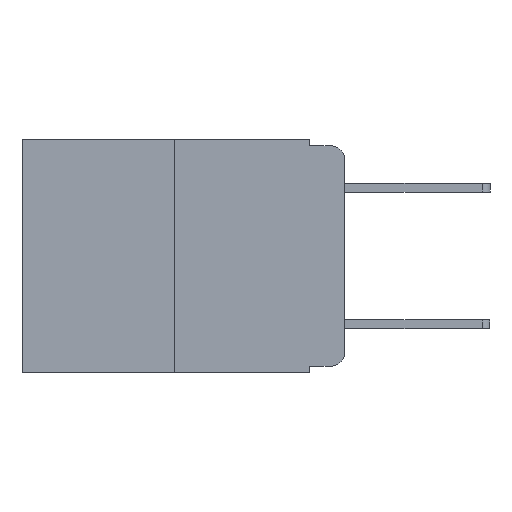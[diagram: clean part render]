
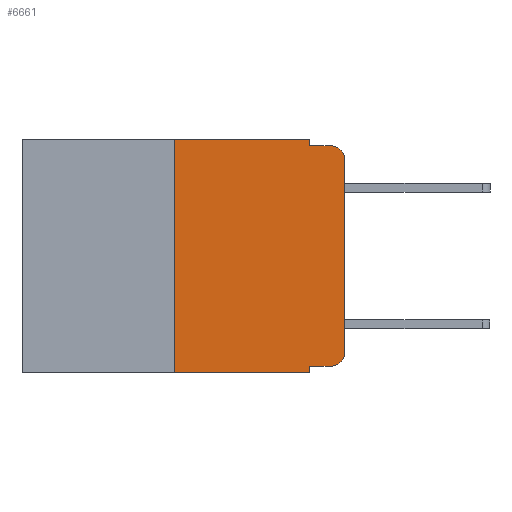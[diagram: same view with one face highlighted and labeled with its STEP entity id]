
A CAD part, left-side view. The second image highlights one B-rep face of the part: STEP entity #6661.
In plain terms, the highlighted planar face has unit normal (-1, 0, 0).
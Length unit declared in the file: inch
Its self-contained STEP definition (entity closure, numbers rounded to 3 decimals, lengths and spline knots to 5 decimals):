
#498 = EDGE_CURVE ( 'NONE', #4194, #19976, #15125, .T. ) ;
#619 = ORIENTED_EDGE ( 'NONE', *, *, #13158, .T. ) ;
#621 = EDGE_CURVE ( 'NONE', #4194, #7882, #17908, .T. ) ;
#713 = CARTESIAN_POINT ( 'NONE',  ( 0., 0.051, -0.01 ) ) ;
#877 = DIRECTION ( 'NONE',  ( 1., 0., 0. ) ) ;
#1221 = CARTESIAN_POINT ( 'NONE',  ( 0., 0.051, -0.343 ) ) ;
#1234 = VECTOR ( 'NONE', #7158, 39.37008 ) ;
#1759 = EDGE_LOOP ( 'NONE', ( #17316, #18535, #5094, #11025, #22263, #22857, #13569, #14815, #619, #7294 ) ) ;
#2315 = VERTEX_POINT ( 'NONE', #12398 ) ;
#2524 = EDGE_CURVE ( 'NONE', #12047, #22004, #4253, .T. ) ;
#2867 = VECTOR ( 'NONE', #16644, 39.37008 ) ;
#3122 = LINE ( 'NONE', #8261, #18510 ) ;
#3480 = DIRECTION ( 'NONE',  ( 0., -1., 0. ) ) ;
#4194 = VERTEX_POINT ( 'NONE', #8887 ) ;
#4246 = VERTEX_POINT ( 'NONE', #22222 ) ;
#4253 = CIRCLE ( 'NONE', #12836, 0.02 ) ;
#4378 = EDGE_CURVE ( 'NONE', #12311, #18752, #13593, .T. ) ;
#5094 = ORIENTED_EDGE ( 'NONE', *, *, #4378, .F. ) ;
#5103 = DIRECTION ( 'NONE',  ( -1., 0., 0. ) ) ;
#5194 = EDGE_CURVE ( 'NONE', #22004, #2315, #16683, .T. ) ;
#5383 = VECTOR ( 'NONE', #17903, 39.37008 ) ;
#5543 = CARTESIAN_POINT ( 'NONE',  ( 0., 0.473, 0. ) ) ;
#6079 = EDGE_CURVE ( 'NONE', #19036, #19976, #25779, .T. ) ;
#6661 = ADVANCED_FACE ( 'NONE', ( #23111 ), #12960, .F. ) ;
#7158 = DIRECTION ( 'NONE',  ( 0., 0., 1. ) ) ;
#7294 = ORIENTED_EDGE ( 'NONE', *, *, #2524, .T. ) ;
#7763 = EDGE_CURVE ( 'NONE', #7882, #4246, #13786, .T. ) ;
#7882 = VERTEX_POINT ( 'NONE', #11914 ) ;
#8009 = CARTESIAN_POINT ( 'NONE',  ( 0., 0.473, -0.343 ) ) ;
#8261 = CARTESIAN_POINT ( 'NONE',  ( 0., 0.051, -0.333 ) ) ;
#8887 = CARTESIAN_POINT ( 'NONE',  ( 0., 0.25, -0.343 ) ) ;
#9467 = CARTESIAN_POINT ( 'NONE',  ( 0., 0.051, -0.333 ) ) ;
#9602 = CARTESIAN_POINT ( 'NONE',  ( 0., 0.051, -0.01 ) ) ;
#9733 = VECTOR ( 'NONE', #19588, 39.37008 ) ;
#9993 = CARTESIAN_POINT ( 'NONE',  ( 0., 0.25, 0. ) ) ;
#10937 = VECTOR ( 'NONE', #14960, 39.37008 ) ;
#11025 = ORIENTED_EDGE ( 'NONE', *, *, #14642, .F. ) ;
#11155 = CARTESIAN_POINT ( 'NONE',  ( 0., 0., -0.313 ) ) ;
#11223 = DIRECTION ( 'NONE',  ( 0., 0., -1. ) ) ;
#11914 = CARTESIAN_POINT ( 'NONE',  ( 0., 0.25, 0. ) ) ;
#12047 = VERTEX_POINT ( 'NONE', #16848 ) ;
#12093 = EDGE_CURVE ( 'NONE', #2315, #18752, #15427, .T. ) ;
#12219 = DIRECTION ( 'NONE',  ( 0., -1., 0. ) ) ;
#12311 = VERTEX_POINT ( 'NONE', #9602 ) ;
#12398 = CARTESIAN_POINT ( 'NONE',  ( 0., 0., -0.03 ) ) ;
#12779 = DIRECTION ( 'NONE',  ( 0., 0., -1. ) ) ;
#12836 = AXIS2_PLACEMENT_3D ( 'NONE', #15555, #18609, #12779 ) ;
#12960 = PLANE ( 'NONE',  #23681 ) ;
#13158 = EDGE_CURVE ( 'NONE', #19036, #12047, #3122, .T. ) ;
#13162 = VECTOR ( 'NONE', #3480, 39.37008 ) ;
#13569 = ORIENTED_EDGE ( 'NONE', *, *, #498, .T. ) ;
#13593 = LINE ( 'NONE', #713, #2867 ) ;
#13786 = LINE ( 'NONE', #5543, #13162 ) ;
#13845 = AXIS2_PLACEMENT_3D ( 'NONE', #17104, #5103, #19094 ) ;
#14642 = EDGE_CURVE ( 'NONE', #4246, #12311, #22182, .T. ) ;
#14815 = ORIENTED_EDGE ( 'NONE', *, *, #6079, .F. ) ;
#14960 = DIRECTION ( 'NONE',  ( 0., 0., -1. ) ) ;
#14984 = DIRECTION ( 'NONE',  ( 0., 0., -1. ) ) ;
#15125 = LINE ( 'NONE', #8009, #9733 ) ;
#15427 = CIRCLE ( 'NONE', #13845, 0.02 ) ;
#15555 = CARTESIAN_POINT ( 'NONE',  ( 0., 0.02, -0.313 ) ) ;
#16644 = DIRECTION ( 'NONE',  ( 0., -1., 0. ) ) ;
#16683 = LINE ( 'NONE', #18020, #5383 ) ;
#16848 = CARTESIAN_POINT ( 'NONE',  ( 0., 0.02, -0.333 ) ) ;
#16915 = CARTESIAN_POINT ( 'NONE',  ( 0., 0.473, 0. ) ) ;
#17104 = CARTESIAN_POINT ( 'NONE',  ( 0., 0.02, -0.03 ) ) ;
#17212 = CARTESIAN_POINT ( 'NONE',  ( 0., 0.051, 0. ) ) ;
#17316 = ORIENTED_EDGE ( 'NONE', *, *, #5194, .T. ) ;
#17903 = DIRECTION ( 'NONE',  ( 0., 0., 1. ) ) ;
#17908 = LINE ( 'NONE', #9993, #1234 ) ;
#18020 = CARTESIAN_POINT ( 'NONE',  ( 0., 0., 0. ) ) ;
#18510 = VECTOR ( 'NONE', #12219, 39.37008 ) ;
#18521 = CARTESIAN_POINT ( 'NONE',  ( 0., 0.02, -0.01 ) ) ;
#18535 = ORIENTED_EDGE ( 'NONE', *, *, #12093, .T. ) ;
#18609 = DIRECTION ( 'NONE',  ( -1., 0., 0. ) ) ;
#18752 = VERTEX_POINT ( 'NONE', #18521 ) ;
#19036 = VERTEX_POINT ( 'NONE', #9467 ) ;
#19094 = DIRECTION ( 'NONE',  ( 0., 0., -1. ) ) ;
#19588 = DIRECTION ( 'NONE',  ( 0., -1., 0. ) ) ;
#19976 = VERTEX_POINT ( 'NONE', #1221 ) ;
#20669 = VECTOR ( 'NONE', #11223, 39.37008 ) ;
#20966 = CARTESIAN_POINT ( 'NONE',  ( 0., 0.051, 0. ) ) ;
#22004 = VERTEX_POINT ( 'NONE', #11155 ) ;
#22182 = LINE ( 'NONE', #20966, #10937 ) ;
#22222 = CARTESIAN_POINT ( 'NONE',  ( 0., 0.051, 0. ) ) ;
#22263 = ORIENTED_EDGE ( 'NONE', *, *, #7763, .F. ) ;
#22857 = ORIENTED_EDGE ( 'NONE', *, *, #621, .F. ) ;
#23111 = FACE_OUTER_BOUND ( 'NONE', #1759, .T. ) ;
#23681 = AXIS2_PLACEMENT_3D ( 'NONE', #16915, #877, #14984 ) ;
#25779 = LINE ( 'NONE', #17212, #20669 ) ;
